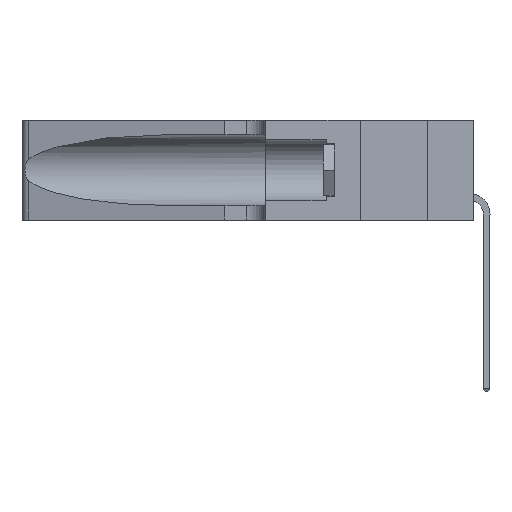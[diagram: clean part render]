
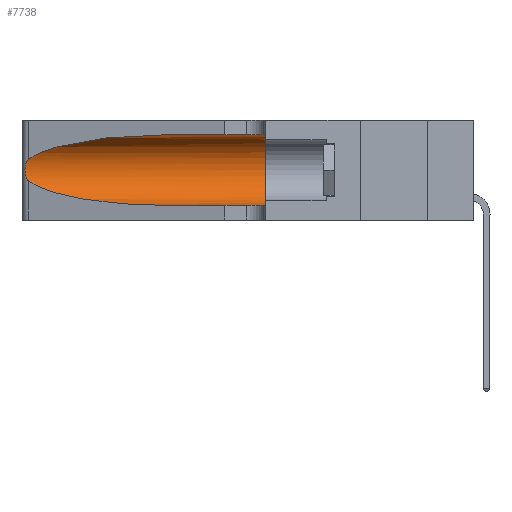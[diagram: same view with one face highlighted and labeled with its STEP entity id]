
A CAD part, left-side view. The second image highlights one B-rep face of the part: STEP entity #7738.
In plain terms, the highlighted cylindrical face has radius 3.308 mm (diameter 6.617 mm), a partial arc.
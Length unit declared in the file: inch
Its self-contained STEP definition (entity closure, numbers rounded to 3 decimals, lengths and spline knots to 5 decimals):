
#167 = CARTESIAN_POINT ( 'NONE',  ( 0.1305, 0.72297, 0.05475 ) ) ;
#454 = CARTESIAN_POINT ( 'NONE',  ( 0.18966, 0.96281, 0.05475 ) ) ;
#1129 = CARTESIAN_POINT ( 'NONE',  ( 0.1305, 0.72297, 0.31525 ) ) ;
#1367 = LINE ( 'NONE', #1799, #8882 ) ;
#1799 = CARTESIAN_POINT ( 'NONE',  ( 0.1305, 1.61858, 0.31525 ) ) ;
#2401 = CARTESIAN_POINT ( 'NONE',  ( 0.25487, 1.22718, 0.14631 ) ) ;
#2737 = CARTESIAN_POINT ( 'NONE',  ( 0.25487, 1.22718, 0.14631 ) ) ;
#2833 = VERTEX_POINT ( 'NONE', #16642 ) ;
#2884 = FACE_OUTER_BOUND ( 'NONE', #21206, .T. ) ;
#4474 = CARTESIAN_POINT ( 'NONE',  ( 0.2373, 1.15595, 0.28018 ) ) ;
#4977 = CARTESIAN_POINT ( 'NONE',  ( 0.1305, 1.61858, 0.185 ) ) ;
#5020 = CARTESIAN_POINT ( 'NONE',  ( 0.25487, 1.22718, 0.14631 ) ) ;
#5484 = VECTOR ( 'NONE', #9302, 39.37008 ) ;
#5942 = CARTESIAN_POINT ( 'NONE',  ( 0.25639, 1.23184, 0.21858 ) ) ;
#6091 = CARTESIAN_POINT ( 'NONE',  ( 0.26075, 1.23896, 0.178 ) ) ;
#6371 = CYLINDRICAL_SURFACE ( 'NONE', #17181, 0.13025 ) ;
#6469 = ORIENTED_EDGE ( 'NONE', *, *, #9448, .T. ) ;
#6837 = DIRECTION ( 'NONE',  ( 0., 0., -1. ) ) ;
#6845 = ORIENTED_EDGE ( 'NONE', *, *, #11463, .F. ) ;
#6994 = DIRECTION ( 'NONE',  ( 0., -1., 0. ) ) ;
#6997 =( BOUNDED_CURVE ( )  B_SPLINE_CURVE ( 3, ( #5020, #18834, #454, #167 ),
 .UNSPECIFIED., .F., .F. ) 
 B_SPLINE_CURVE_WITH_KNOTS ( ( 4, 4 ),
 ( 3.44316, 4.71239 ),
 .UNSPECIFIED. ) 
 CURVE ( )  GEOMETRIC_REPRESENTATION_ITEM ( )  RATIONAL_B_SPLINE_CURVE ( ( 1., 0.87, 0.87, 1. ) ) 
 REPRESENTATION_ITEM ( '' )  );
#7428 = CARTESIAN_POINT ( 'NONE',  ( 0.1305, 1.61858, 0.05475 ) ) ;
#7487 = CARTESIAN_POINT ( 'NONE',  ( 0.1305, 0.35, 0.05475 ) ) ;
#7504 = CARTESIAN_POINT ( 'NONE',  ( 0.25555, 1.22994, 0.2215 ) ) ;
#7577 = CARTESIAN_POINT ( 'NONE',  ( 0.25787, 1.23484, 0.2124 ) ) ;
#7618 = CARTESIAN_POINT ( 'NONE',  ( 0.1305, 0.72297, 0.31525 ) ) ;
#7654 = CARTESIAN_POINT ( 'NONE',  ( 0.25856, 1.23593, 0.16098 ) ) ;
#7726 = CARTESIAN_POINT ( 'NONE',  ( 0.26018, 1.23835, 0.19895 ) ) ;
#7738 = ADVANCED_FACE ( 'NONE', ( #2884 ), #6371, .F. ) ;
#8102 = ORIENTED_EDGE ( 'NONE', *, *, #13849, .T. ) ;
#8476 = AXIS2_PLACEMENT_3D ( 'NONE', #13265, #16848, #11474 ) ;
#8882 = VECTOR ( 'NONE', #6994, 39.37008 ) ;
#9302 = DIRECTION ( 'NONE',  ( 0., -1., 0. ) ) ;
#9448 = EDGE_CURVE ( 'NONE', #2833, #16144, #20804, .T. ) ;
#9803 = VERTEX_POINT ( 'NONE', #7618 ) ;
#10215 = DIRECTION ( 'NONE',  ( 0., -1., 0. ) ) ;
#11224 = CARTESIAN_POINT ( 'NONE',  ( 0.25555, 1.22993, 0.14849 ) ) ;
#11463 = EDGE_CURVE ( 'NONE', #15122, #16144, #19941, .T. ) ;
#11474 = DIRECTION ( 'NONE',  ( 0., 0., 1. ) ) ;
#11524 = EDGE_CURVE ( 'NONE', #9803, #15122, #1367, .T. ) ;
#12648 = CARTESIAN_POINT ( 'NONE',  ( 0.25854, 1.2359, 0.20912 ) ) ;
#13019 = EDGE_CURVE ( 'NONE', #16988, #2833, #6997, .T. ) ;
#13047 = CARTESIAN_POINT ( 'NONE',  ( 0.1305, 0.35, 0.31525 ) ) ;
#13265 = CARTESIAN_POINT ( 'NONE',  ( 0.1305, 0.35, 0.185 ) ) ;
#13650 = VERTEX_POINT ( 'NONE', #17364 ) ;
#13849 = EDGE_CURVE ( 'NONE', #13650, #16988, #18709, .T. ) ;
#14684 =( BOUNDED_CURVE ( )  B_SPLINE_CURVE ( 3, ( #1129, #20178, #4474, #15046 ),
 .UNSPECIFIED., .F., .F. ) 
 B_SPLINE_CURVE_WITH_KNOTS ( ( 4, 4 ),
 ( 1.5708, 2.84003 ),
 .UNSPECIFIED. ) 
 CURVE ( )  GEOMETRIC_REPRESENTATION_ITEM ( )  RATIONAL_B_SPLINE_CURVE ( ( 1., 0.87, 0.87, 1. ) ) 
 REPRESENTATION_ITEM ( '' )  );
#15046 = CARTESIAN_POINT ( 'NONE',  ( 0.25487, 1.22718, 0.22369 ) ) ;
#15076 = ORIENTED_EDGE ( 'NONE', *, *, #11524, .F. ) ;
#15122 = VERTEX_POINT ( 'NONE', #13047 ) ;
#15164 = ORIENTED_EDGE ( 'NONE', *, *, #13019, .T. ) ;
#15855 = CARTESIAN_POINT ( 'NONE',  ( 0.25487, 1.22718, 0.22369 ) ) ;
#16144 = VERTEX_POINT ( 'NONE', #7487 ) ;
#16384 = CARTESIAN_POINT ( 'NONE',  ( 0.26075, 1.23896, 0.19203 ) ) ;
#16642 = CARTESIAN_POINT ( 'NONE',  ( 0.1305, 0.72297, 0.05475 ) ) ;
#16848 = DIRECTION ( 'NONE',  ( 0., 1., 0. ) ) ;
#16988 = VERTEX_POINT ( 'NONE', #2737 ) ;
#17181 = AXIS2_PLACEMENT_3D ( 'NONE', #4977, #10215, #6837 ) ;
#17364 = CARTESIAN_POINT ( 'NONE',  ( 0.25487, 1.22718, 0.22369 ) ) ;
#18709 = B_SPLINE_CURVE_WITH_KNOTS ( 'NONE', 3,
 ( #15855, #7504, #5942, #7577, #12648, #7726, #16384, #6091, #21552, #7654, #19686, #19837, #11224, #2401 ),
 .UNSPECIFIED., .F., .F.,
 ( 4, 2, 2, 2, 2, 2, 4 ),
 ( 0., 0.00027, 0.00053, 0.00107, 0.0016, 0.00187, 0.00214 ),
 .UNSPECIFIED. ) ;
#18834 = CARTESIAN_POINT ( 'NONE',  ( 0.2373, 1.15595, 0.08982 ) ) ;
#19423 = EDGE_CURVE ( 'NONE', #9803, #13650, #14684, .T. ) ;
#19626 = ORIENTED_EDGE ( 'NONE', *, *, #19423, .T. ) ;
#19686 = CARTESIAN_POINT ( 'NONE',  ( 0.25789, 1.23486, 0.15765 ) ) ;
#19837 = CARTESIAN_POINT ( 'NONE',  ( 0.25639, 1.23186, 0.15144 ) ) ;
#19941 = CIRCLE ( 'NONE', #8476, 0.13025 ) ;
#20178 = CARTESIAN_POINT ( 'NONE',  ( 0.18966, 0.96281, 0.31525 ) ) ;
#20804 = LINE ( 'NONE', #7428, #5484 ) ;
#21206 = EDGE_LOOP ( 'NONE', ( #19626, #8102, #15164, #6469, #6845, #15076 ) ) ;
#21552 = CARTESIAN_POINT ( 'NONE',  ( 0.26017, 1.23833, 0.17102 ) ) ;
